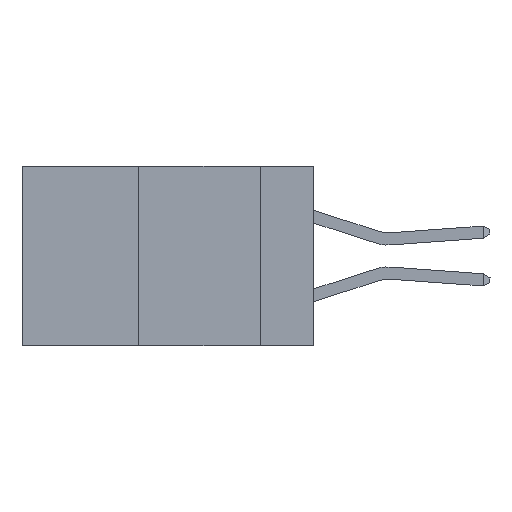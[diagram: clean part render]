
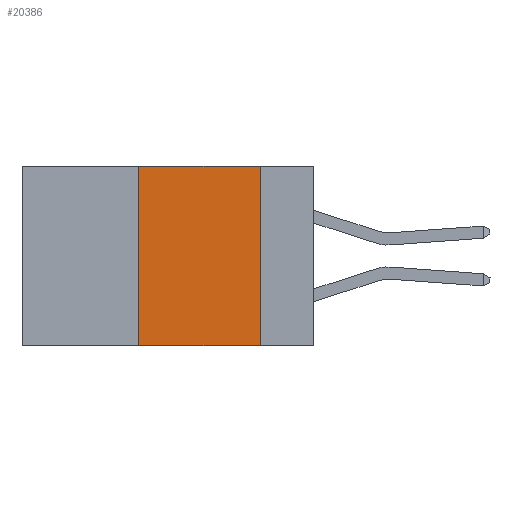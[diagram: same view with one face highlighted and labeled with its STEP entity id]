
A CAD part, left-side view. The second image highlights one B-rep face of the part: STEP entity #20386.
In plain terms, the highlighted planar face has unit normal (-1, 0, 0).
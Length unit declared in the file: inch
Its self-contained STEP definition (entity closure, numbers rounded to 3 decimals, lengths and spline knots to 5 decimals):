
#104 = CARTESIAN_POINT ( 'NONE',  ( 0., 0.6, 0. ) ) ;
#133 = VERTEX_POINT ( 'NONE', #24575 ) ;
#1982 = DIRECTION ( 'NONE',  ( 0., 0., -1. ) ) ;
#2191 = PLANE ( 'NONE',  #18443 ) ;
#2275 = CARTESIAN_POINT ( 'NONE',  ( 0., 0.36, 0. ) ) ;
#2753 = VERTEX_POINT ( 'NONE', #20065 ) ;
#3830 = DIRECTION ( 'NONE',  ( 0., 0., 1. ) ) ;
#5468 = VECTOR ( 'NONE', #12138, 39.37008 ) ;
#5623 = CARTESIAN_POINT ( 'NONE',  ( 0., 0.36, 0. ) ) ;
#6428 = CARTESIAN_POINT ( 'NONE',  ( 0., 0.6, 0. ) ) ;
#6476 = CARTESIAN_POINT ( 'NONE',  ( 0., 0.11, 0. ) ) ;
#7289 = VERTEX_POINT ( 'NONE', #14406 ) ;
#8673 = DIRECTION ( 'NONE',  ( 1., 0., 0. ) ) ;
#9492 = VERTEX_POINT ( 'NONE', #5623 ) ;
#10793 = LINE ( 'NONE', #6428, #5468 ) ;
#12138 = DIRECTION ( 'NONE',  ( 0., -1., 0. ) ) ;
#12630 = LINE ( 'NONE', #21222, #13944 ) ;
#13923 = ORIENTED_EDGE ( 'NONE', *, *, #26007, .F. ) ;
#13944 = VECTOR ( 'NONE', #16686, 39.37008 ) ;
#14406 = CARTESIAN_POINT ( 'NONE',  ( 0., 0.11, 0. ) ) ;
#14792 = EDGE_LOOP ( 'NONE', ( #22211, #17868, #13923, #24588 ) ) ;
#16686 = DIRECTION ( 'NONE',  ( 0., -1., 0. ) ) ;
#17868 = ORIENTED_EDGE ( 'NONE', *, *, #21589, .F. ) ;
#18057 = EDGE_CURVE ( 'NONE', #7289, #2753, #23220, .T. ) ;
#18443 = AXIS2_PLACEMENT_3D ( 'NONE', #104, #8673, #23440 ) ;
#19088 = FACE_OUTER_BOUND ( 'NONE', #14792, .T. ) ;
#20065 = CARTESIAN_POINT ( 'NONE',  ( 0., 0.11, -0.37 ) ) ;
#20328 = EDGE_CURVE ( 'NONE', #133, #2753, #12630, .T. ) ;
#20386 = ADVANCED_FACE ( 'NONE', ( #19088 ), #2191, .F. ) ;
#21222 = CARTESIAN_POINT ( 'NONE',  ( 0., 0.6, -0.37 ) ) ;
#21573 = LINE ( 'NONE', #2275, #26290 ) ;
#21589 = EDGE_CURVE ( 'NONE', #9492, #7289, #10793, .T. ) ;
#22211 = ORIENTED_EDGE ( 'NONE', *, *, #18057, .F. ) ;
#23220 = LINE ( 'NONE', #6476, #25616 ) ;
#23440 = DIRECTION ( 'NONE',  ( 0., 0., -1. ) ) ;
#24575 = CARTESIAN_POINT ( 'NONE',  ( 0., 0.36, -0.37 ) ) ;
#24588 = ORIENTED_EDGE ( 'NONE', *, *, #20328, .T. ) ;
#25616 = VECTOR ( 'NONE', #1982, 39.37008 ) ;
#26007 = EDGE_CURVE ( 'NONE', #133, #9492, #21573, .T. ) ;
#26290 = VECTOR ( 'NONE', #3830, 39.37008 ) ;
